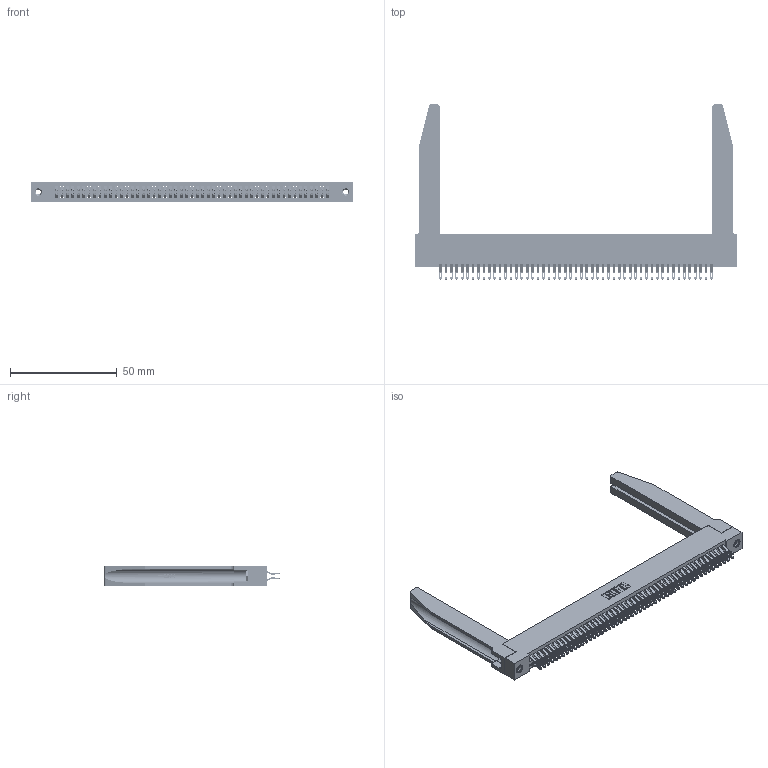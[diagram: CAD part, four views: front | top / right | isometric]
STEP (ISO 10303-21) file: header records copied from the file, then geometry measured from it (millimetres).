
FILE_DESCRIPTION (( 'STEP AP203' ), '1' );
FILE_NAME ('395-102-555-278.STEP', '2019-10-26T18:52:29', ( '' ), ( '' ), 'SwSTEP 2.0', 'SolidWorks 2016', '' );
FILE_SCHEMA (( 'CONFIG_CONTROL_DESIGN' ));
Length unit declared in the file: inch
Products named in the file (5): 395-102-555-278; 345 Part_Flush Mounting Lugs - 0.156 Dia-TH; 345-292-001_555 Tail; 345-250-001_345-250-001-102; 345-220-078_345-220-078
Assembly tree (107 placements, depth 2):
  395-102-555-278
    345 Part_Flush Mounting Lugs - 0.156 Dia-TH
    345-292-001_555 Tail  x102
    345-250-001_345-250-001-102  x2
    345-220-078_345-220-078  x2
Bounding box: 150.77 x 82.09 x 9.4 mm (x, y, z)
Volume: 22796.2 mm3; surface area: 30252.4 mm2
Topology: 107 solids, 107 shells, 6072 faces, 19003 edges, 12658 vertices
Faces by surface type: plane 3384, cylinder 2636, bspline 36, cone 12, torus 4
Entity records: 43870 total; most frequent: CARTESIAN_POINT 8297, ORIENTED_EDGE 7098, DIRECTION 6267, EDGE_CURVE 3549, LINE 3099, VECTOR 3099, VERTEX_POINT 2360, AXIS2_PLACEMENT_3D 1584
